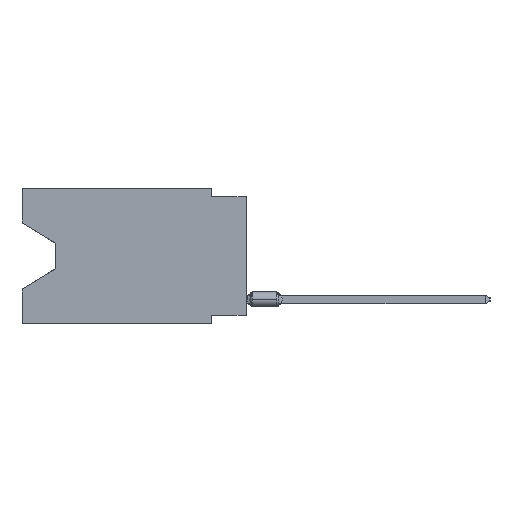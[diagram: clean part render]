
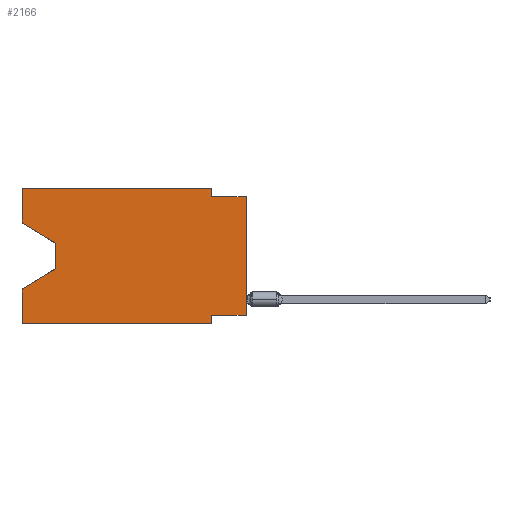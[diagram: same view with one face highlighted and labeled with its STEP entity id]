
A CAD part, left-side view. The second image highlights one B-rep face of the part: STEP entity #2166.
In plain terms, the highlighted planar face has unit normal (-1, 0, 0).
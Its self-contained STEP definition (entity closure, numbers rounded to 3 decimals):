
#622 = EDGE_CURVE ( 'NONE', #24294, #14341, #19994, .T. ) ;
#1115 = CARTESIAN_POINT ( 'NONE',  ( 0., 2.54, -0.635 ) ) ;
#1794 = DIRECTION ( 'NONE',  ( 0., 1., 0. ) ) ;
#2166 = ADVANCED_FACE ( 'NONE', ( #3679 ), #27691, .F. ) ;
#2590 = ORIENTED_EDGE ( 'NONE', *, *, #6194, .F. ) ;
#2796 = VECTOR ( 'NONE', #44099, 1000. ) ;
#3340 = DIRECTION ( 'NONE',  ( 0., 0., 1. ) ) ;
#3531 = EDGE_CURVE ( 'NONE', #43724, #9739, #40650, .T. ) ;
#3679 = FACE_OUTER_BOUND ( 'NONE', #41849, .T. ) ;
#4731 = CARTESIAN_POINT ( 'NONE',  ( 0., 16.383, 0. ) ) ;
#5285 = EDGE_CURVE ( 'NONE', #38314, #45098, #21112, .T. ) ;
#5312 = CARTESIAN_POINT ( 'NONE',  ( 0., 2.54, -9.271 ) ) ;
#5459 = ORIENTED_EDGE ( 'NONE', *, *, #31252, .F. ) ;
#5515 = CARTESIAN_POINT ( 'NONE',  ( 0., 16.383, 0. ) ) ;
#5793 = EDGE_CURVE ( 'NONE', #22713, #45098, #6346, .T. ) ;
#6194 = EDGE_CURVE ( 'NONE', #9739, #28335, #35629, .T. ) ;
#6291 = LINE ( 'NONE', #37970, #35484 ) ;
#6346 = LINE ( 'NONE', #37803, #38511 ) ;
#6990 = CARTESIAN_POINT ( 'NONE',  ( 0., 0., -0.635 ) ) ;
#7265 = LINE ( 'NONE', #4731, #8357 ) ;
#8357 = VECTOR ( 'NONE', #28741, 1000. ) ;
#8544 = CARTESIAN_POINT ( 'NONE',  ( 0., 0., 0. ) ) ;
#8770 = DIRECTION ( 'NONE',  ( 0., 0., 1. ) ) ;
#9460 = ORIENTED_EDGE ( 'NONE', *, *, #42700, .T. ) ;
#9739 = VERTEX_POINT ( 'NONE', #38782 ) ;
#9966 = VECTOR ( 'NONE', #44363, 1000. ) ;
#10109 = VERTEX_POINT ( 'NONE', #6990 ) ;
#10651 = DIRECTION ( 'NONE',  ( 0., 0., -1. ) ) ;
#10675 = VECTOR ( 'NONE', #3340, 1000. ) ;
#10812 = DIRECTION ( 'NONE',  ( 0., 0., -1. ) ) ;
#11481 = ORIENTED_EDGE ( 'NONE', *, *, #5793, .F. ) ;
#12042 = CARTESIAN_POINT ( 'NONE',  ( 0., 16.383, 0. ) ) ;
#12078 = EDGE_CURVE ( 'NONE', #19901, #41922, #35288, .T. ) ;
#13184 = VECTOR ( 'NONE', #8770, 1000. ) ;
#14341 = VERTEX_POINT ( 'NONE', #31619 ) ;
#14508 = ORIENTED_EDGE ( 'NONE', *, *, #5285, .T. ) ;
#16271 = ORIENTED_EDGE ( 'NONE', *, *, #41138, .F. ) ;
#16541 = CARTESIAN_POINT ( 'NONE',  ( 0., 16.383, -2.546 ) ) ;
#16704 = VECTOR ( 'NONE', #25541, 1000. ) ;
#16745 = DIRECTION ( 'NONE',  ( 0., 0., -1. ) ) ;
#17418 = CARTESIAN_POINT ( 'NONE',  ( 0., 16.383, 0. ) ) ;
#17531 = DIRECTION ( 'NONE',  ( 1., 0., 0. ) ) ;
#18194 = LINE ( 'NONE', #41063, #20643 ) ;
#18277 = CARTESIAN_POINT ( 'NONE',  ( 0., 2.54, 0. ) ) ;
#18543 = CARTESIAN_POINT ( 'NONE',  ( 0., 16.383, -2.546 ) ) ;
#18922 = AXIS2_PLACEMENT_3D ( 'NONE', #21224, #17531, #10812 ) ;
#19511 = CARTESIAN_POINT ( 'NONE',  ( 0., 16.383, -7.36 ) ) ;
#19901 = VERTEX_POINT ( 'NONE', #37176 ) ;
#19994 = LINE ( 'NONE', #16541, #39882 ) ;
#20183 = ORIENTED_EDGE ( 'NONE', *, *, #21075, .F. ) ;
#20643 = VECTOR ( 'NONE', #1794, 1000. ) ;
#21075 = EDGE_CURVE ( 'NONE', #41385, #22713, #18194, .T. ) ;
#21112 = LINE ( 'NONE', #25258, #38360 ) ;
#21224 = CARTESIAN_POINT ( 'NONE',  ( 0., 16.383, 0. ) ) ;
#22713 = VERTEX_POINT ( 'NONE', #5312 ) ;
#24294 = VERTEX_POINT ( 'NONE', #18543 ) ;
#24847 = CARTESIAN_POINT ( 'NONE',  ( 0., 13.97, -5.893 ) ) ;
#25258 = CARTESIAN_POINT ( 'NONE',  ( 0., 16.383, -9.906 ) ) ;
#25541 = DIRECTION ( 'NONE',  ( 0., 0.855, -0.519 ) ) ;
#25972 = ORIENTED_EDGE ( 'NONE', *, *, #3531, .F. ) ;
#26391 = ORIENTED_EDGE ( 'NONE', *, *, #33236, .F. ) ;
#27691 = PLANE ( 'NONE',  #18922 ) ;
#28261 = LINE ( 'NONE', #17418, #10675 ) ;
#28335 = VERTEX_POINT ( 'NONE', #1115 ) ;
#28741 = DIRECTION ( 'NONE',  ( 0., 0., 1. ) ) ;
#28887 = VECTOR ( 'NONE', #32373, 1000. ) ;
#29480 = CARTESIAN_POINT ( 'NONE',  ( 0., 16.383, -9.906 ) ) ;
#31252 = EDGE_CURVE ( 'NONE', #24294, #43724, #7265, .T. ) ;
#31619 = CARTESIAN_POINT ( 'NONE',  ( 0., 13.97, -4.013 ) ) ;
#32373 = DIRECTION ( 'NONE',  ( 0., 0., -1. ) ) ;
#32999 = CARTESIAN_POINT ( 'NONE',  ( 0., 0., -9.271 ) ) ;
#33236 = EDGE_CURVE ( 'NONE', #38314, #41922, #28261, .T. ) ;
#33507 = ORIENTED_EDGE ( 'NONE', *, *, #622, .T. ) ;
#33715 = CARTESIAN_POINT ( 'NONE',  ( 0., 0., -0.635 ) ) ;
#34409 = LINE ( 'NONE', #33715, #9966 ) ;
#35288 = LINE ( 'NONE', #24847, #16704 ) ;
#35484 = VECTOR ( 'NONE', #10651, 1000. ) ;
#35629 = LINE ( 'NONE', #18277, #28887 ) ;
#37176 = CARTESIAN_POINT ( 'NONE',  ( 0., 13.97, -5.893 ) ) ;
#37803 = CARTESIAN_POINT ( 'NONE',  ( 0., 2.54, -9.906 ) ) ;
#37970 = CARTESIAN_POINT ( 'NONE',  ( 0., 13.97, -4.013 ) ) ;
#38314 = VERTEX_POINT ( 'NONE', #29480 ) ;
#38360 = VECTOR ( 'NONE', #39400, 1000. ) ;
#38511 = VECTOR ( 'NONE', #16745, 1000. ) ;
#38782 = CARTESIAN_POINT ( 'NONE',  ( 0., 2.54, 0. ) ) ;
#39400 = DIRECTION ( 'NONE',  ( 0., -1., 0. ) ) ;
#39882 = VECTOR ( 'NONE', #41270, 1000. ) ;
#40229 = LINE ( 'NONE', #8544, #13184 ) ;
#40650 = LINE ( 'NONE', #5515, #2796 ) ;
#41063 = CARTESIAN_POINT ( 'NONE',  ( 0., 0., -9.271 ) ) ;
#41138 = EDGE_CURVE ( 'NONE', #28335, #10109, #34409, .T. ) ;
#41270 = DIRECTION ( 'NONE',  ( 0., -0.855, -0.519 ) ) ;
#41385 = VERTEX_POINT ( 'NONE', #32999 ) ;
#41564 = ORIENTED_EDGE ( 'NONE', *, *, #43450, .T. ) ;
#41849 = EDGE_LOOP ( 'NONE', ( #33507, #41564, #44751, #26391, #14508, #11481, #20183, #9460, #16271, #2590, #25972, #5459 ) ) ;
#41922 = VERTEX_POINT ( 'NONE', #19511 ) ;
#42700 = EDGE_CURVE ( 'NONE', #41385, #10109, #40229, .T. ) ;
#43450 = EDGE_CURVE ( 'NONE', #14341, #19901, #6291, .T. ) ;
#43724 = VERTEX_POINT ( 'NONE', #12042 ) ;
#44099 = DIRECTION ( 'NONE',  ( 0., -1., 0. ) ) ;
#44363 = DIRECTION ( 'NONE',  ( 0., -1., 0. ) ) ;
#44751 = ORIENTED_EDGE ( 'NONE', *, *, #12078, .T. ) ;
#45098 = VERTEX_POINT ( 'NONE', #45311 ) ;
#45311 = CARTESIAN_POINT ( 'NONE',  ( 0., 2.54, -9.906 ) ) ;
